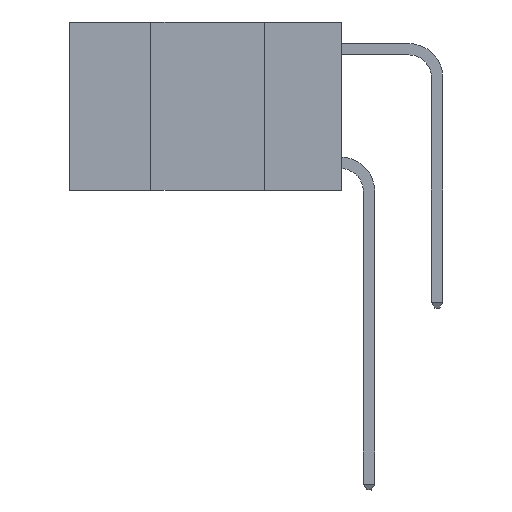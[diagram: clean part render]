
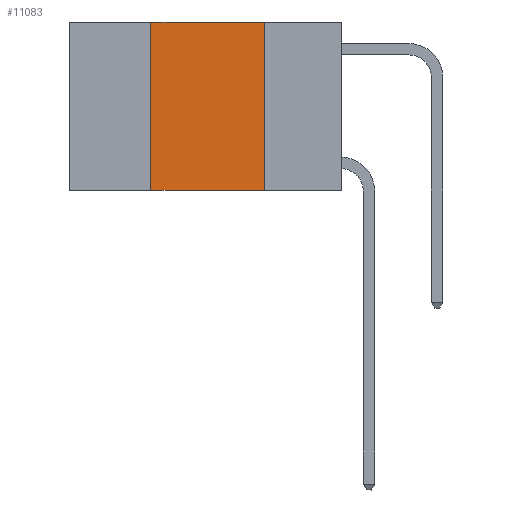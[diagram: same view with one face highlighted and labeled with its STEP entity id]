
A CAD part, left-side view. The second image highlights one B-rep face of the part: STEP entity #11083.
In plain terms, the highlighted planar face has unit normal (-1, 0, 0).
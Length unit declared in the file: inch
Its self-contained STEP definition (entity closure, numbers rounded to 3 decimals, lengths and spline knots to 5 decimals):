
#641 = CARTESIAN_POINT ( 'NONE',  ( 0., 0.17, 0. ) ) ;
#891 = ORIENTED_EDGE ( 'NONE', *, *, #16094, .F. ) ;
#1059 = EDGE_CURVE ( 'NONE', #12221, #1502, #10992, .T. ) ;
#1430 = ORIENTED_EDGE ( 'NONE', *, *, #10294, .F. ) ;
#1502 = VERTEX_POINT ( 'NONE', #6565 ) ;
#2103 = CARTESIAN_POINT ( 'NONE',  ( 0., 0.17, -0.37 ) ) ;
#2214 = EDGE_CURVE ( 'NONE', #12221, #9383, #11202, .T. ) ;
#3008 = DIRECTION ( 'NONE',  ( 0., 0., -1. ) ) ;
#3061 = ORIENTED_EDGE ( 'NONE', *, *, #1059, .F. ) ;
#3403 = CARTESIAN_POINT ( 'NONE',  ( 0., 0.6, -0.37 ) ) ;
#3778 = CARTESIAN_POINT ( 'NONE',  ( 0., 0.42, 0. ) ) ;
#4661 = DIRECTION ( 'NONE',  ( 0., -1., 0. ) ) ;
#5519 = EDGE_LOOP ( 'NONE', ( #891, #1430, #3061, #5938 ) ) ;
#5540 = PLANE ( 'NONE',  #21121 ) ;
#5672 = LINE ( 'NONE', #14701, #14578 ) ;
#5938 = ORIENTED_EDGE ( 'NONE', *, *, #2214, .T. ) ;
#6346 = DIRECTION ( 'NONE',  ( 0., 0., 1. ) ) ;
#6565 = CARTESIAN_POINT ( 'NONE',  ( 0., 0.42, 0. ) ) ;
#6653 = CARTESIAN_POINT ( 'NONE',  ( 0., 0.42, -0.37 ) ) ;
#7203 = DIRECTION ( 'NONE',  ( 0., 0., -1. ) ) ;
#9383 = VERTEX_POINT ( 'NONE', #2103 ) ;
#9678 = CARTESIAN_POINT ( 'NONE',  ( 0., 0.6, 0. ) ) ;
#10045 = VERTEX_POINT ( 'NONE', #641 ) ;
#10294 = EDGE_CURVE ( 'NONE', #1502, #10045, #10577, .T. ) ;
#10474 = VECTOR ( 'NONE', #6346, 39.37008 ) ;
#10577 = LINE ( 'NONE', #9678, #19382 ) ;
#10992 = LINE ( 'NONE', #3778, #10474 ) ;
#11083 = ADVANCED_FACE ( 'NONE', ( #13464 ), #5540, .F. ) ;
#11202 = LINE ( 'NONE', #3403, #15661 ) ;
#11720 = DIRECTION ( 'NONE',  ( 0., -1., 0. ) ) ;
#12221 = VERTEX_POINT ( 'NONE', #6653 ) ;
#13464 = FACE_OUTER_BOUND ( 'NONE', #5519, .T. ) ;
#14578 = VECTOR ( 'NONE', #3008, 39.37008 ) ;
#14701 = CARTESIAN_POINT ( 'NONE',  ( 0., 0.17, 0. ) ) ;
#15661 = VECTOR ( 'NONE', #11720, 39.37008 ) ;
#16094 = EDGE_CURVE ( 'NONE', #10045, #9383, #5672, .T. ) ;
#17133 = CARTESIAN_POINT ( 'NONE',  ( 0., 0.6, 0. ) ) ;
#17202 = DIRECTION ( 'NONE',  ( 1., 0., 0. ) ) ;
#19382 = VECTOR ( 'NONE', #4661, 39.37008 ) ;
#21121 = AXIS2_PLACEMENT_3D ( 'NONE', #17133, #17202, #7203 ) ;
